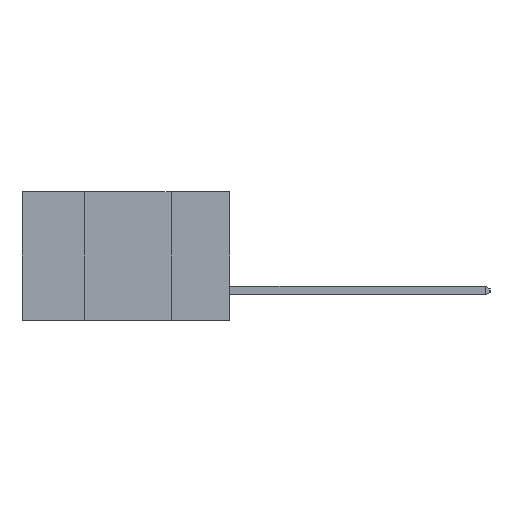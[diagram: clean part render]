
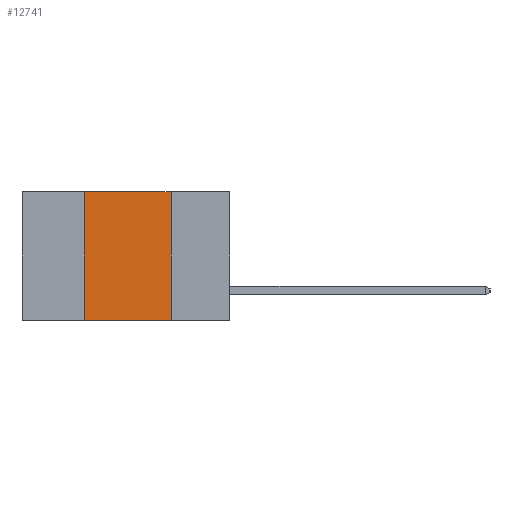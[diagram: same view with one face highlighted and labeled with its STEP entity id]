
A CAD part, left-side view. The second image highlights one B-rep face of the part: STEP entity #12741.
In plain terms, the highlighted planar face has unit normal (-1, 0, 0).
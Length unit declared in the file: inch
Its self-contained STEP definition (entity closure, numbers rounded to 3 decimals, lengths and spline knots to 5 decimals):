
#1045 = CARTESIAN_POINT ( 'NONE',  ( 0., 0.6, 0. ) ) ;
#1410 = CARTESIAN_POINT ( 'NONE',  ( 0., 0.17, 0. ) ) ;
#1411 = VECTOR ( 'NONE', #5324, 39.37008 ) ;
#1660 = FACE_OUTER_BOUND ( 'NONE', #17623, .T. ) ;
#2030 = VECTOR ( 'NONE', #17142, 39.37008 ) ;
#2439 = DIRECTION ( 'NONE',  ( 0., 0., -1. ) ) ;
#2587 = VERTEX_POINT ( 'NONE', #4899 ) ;
#4807 = LINE ( 'NONE', #1410, #11650 ) ;
#4899 = CARTESIAN_POINT ( 'NONE',  ( 0., 0.17, 0. ) ) ;
#5041 = ORIENTED_EDGE ( 'NONE', *, *, #14998, .F. ) ;
#5160 = PLANE ( 'NONE',  #9895 ) ;
#5222 = VERTEX_POINT ( 'NONE', #14642 ) ;
#5324 = DIRECTION ( 'NONE',  ( 0., -1., 0. ) ) ;
#7279 = CARTESIAN_POINT ( 'NONE',  ( 0., 0.17, -0.37 ) ) ;
#8153 = VECTOR ( 'NONE', #13072, 39.37008 ) ;
#9133 = CARTESIAN_POINT ( 'NONE',  ( 0., 0.42, 0. ) ) ;
#9154 = ORIENTED_EDGE ( 'NONE', *, *, #14105, .F. ) ;
#9390 = LINE ( 'NONE', #9133, #2030 ) ;
#9453 = EDGE_CURVE ( 'NONE', #5222, #2587, #15260, .T. ) ;
#9537 = CARTESIAN_POINT ( 'NONE',  ( 0., 0.42, -0.37 ) ) ;
#9655 = EDGE_CURVE ( 'NONE', #11088, #9903, #15464, .T. ) ;
#9895 = AXIS2_PLACEMENT_3D ( 'NONE', #1045, #10695, #2439 ) ;
#9903 = VERTEX_POINT ( 'NONE', #7279 ) ;
#10695 = DIRECTION ( 'NONE',  ( 1., 0., 0. ) ) ;
#11040 = DIRECTION ( 'NONE',  ( 0., 0., -1. ) ) ;
#11088 = VERTEX_POINT ( 'NONE', #9537 ) ;
#11650 = VECTOR ( 'NONE', #11040, 39.37008 ) ;
#12741 = ADVANCED_FACE ( 'NONE', ( #1660 ), #5160, .F. ) ;
#13072 = DIRECTION ( 'NONE',  ( 0., -1., 0. ) ) ;
#14105 = EDGE_CURVE ( 'NONE', #11088, #5222, #9390, .T. ) ;
#14642 = CARTESIAN_POINT ( 'NONE',  ( 0., 0.42, 0. ) ) ;
#14798 = CARTESIAN_POINT ( 'NONE',  ( 0., 0.6, -0.37 ) ) ;
#14998 = EDGE_CURVE ( 'NONE', #2587, #9903, #4807, .T. ) ;
#15260 = LINE ( 'NONE', #17109, #8153 ) ;
#15464 = LINE ( 'NONE', #14798, #1411 ) ;
#15838 = ORIENTED_EDGE ( 'NONE', *, *, #9453, .F. ) ;
#17109 = CARTESIAN_POINT ( 'NONE',  ( 0., 0.6, 0. ) ) ;
#17112 = ORIENTED_EDGE ( 'NONE', *, *, #9655, .T. ) ;
#17142 = DIRECTION ( 'NONE',  ( 0., 0., 1. ) ) ;
#17623 = EDGE_LOOP ( 'NONE', ( #5041, #15838, #9154, #17112 ) ) ;
